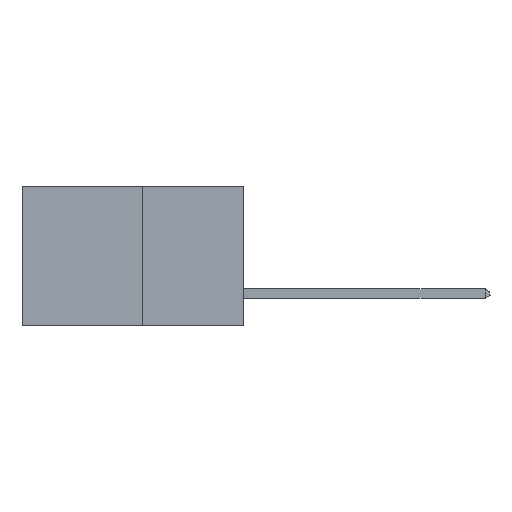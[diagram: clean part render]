
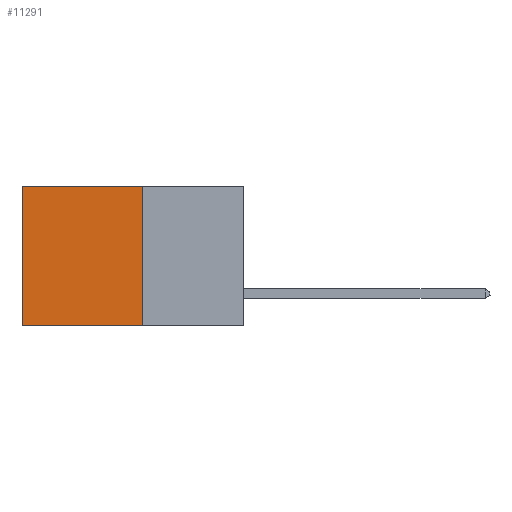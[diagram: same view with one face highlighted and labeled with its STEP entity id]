
A CAD part, left-side view. The second image highlights one B-rep face of the part: STEP entity #11291.
In plain terms, the highlighted planar face has unit normal (-1, 0, 0).
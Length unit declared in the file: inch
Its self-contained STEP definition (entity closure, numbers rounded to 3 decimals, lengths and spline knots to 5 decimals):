
#243 = ORIENTED_EDGE ( 'NONE', *, *, #28271, .T. ) ;
#810 = EDGE_CURVE ( 'NONE', #20137, #5224, #26072, .T. ) ;
#2135 = FACE_OUTER_BOUND ( 'NONE', #20088, .T. ) ;
#4291 = DIRECTION ( 'NONE',  ( 0., 1., 0. ) ) ;
#4607 = ORIENTED_EDGE ( 'NONE', *, *, #16943, .F. ) ;
#5224 = VERTEX_POINT ( 'NONE', #22980 ) ;
#7278 = CARTESIAN_POINT ( 'NONE',  ( 0.277, 0.27, -0.37 ) ) ;
#7582 = CARTESIAN_POINT ( 'NONE',  ( 0.277, 0.59, -0.37 ) ) ;
#8213 = VECTOR ( 'NONE', #23368, 39.37008 ) ;
#8391 = CARTESIAN_POINT ( 'NONE',  ( 0.277, 0.59, -0.37 ) ) ;
#9512 = DIRECTION ( 'NONE',  ( 0., 0., -1. ) ) ;
#9771 = VERTEX_POINT ( 'NONE', #8391 ) ;
#10930 = CARTESIAN_POINT ( 'NONE',  ( 0.277, 0.27, 0. ) ) ;
#11291 = ADVANCED_FACE ( 'NONE', ( #2135 ), #18422, .F. ) ;
#11837 = CARTESIAN_POINT ( 'NONE',  ( 0.277, 0.59, 0. ) ) ;
#14369 = ORIENTED_EDGE ( 'NONE', *, *, #810, .F. ) ;
#15660 = VERTEX_POINT ( 'NONE', #11837 ) ;
#16943 = EDGE_CURVE ( 'NONE', #5224, #9771, #26947, .T. ) ;
#16952 = CARTESIAN_POINT ( 'NONE',  ( 0.277, 0.27, 0. ) ) ;
#18422 = PLANE ( 'NONE',  #28619 ) ;
#18614 = CARTESIAN_POINT ( 'NONE',  ( 0.277, 0.27, -0.37 ) ) ;
#20004 = VECTOR ( 'NONE', #20969, 39.37008 ) ;
#20088 = EDGE_LOOP ( 'NONE', ( #243, #4607, #14369, #20674 ) ) ;
#20137 = VERTEX_POINT ( 'NONE', #16952 ) ;
#20281 = VECTOR ( 'NONE', #27569, 39.37008 ) ;
#20674 = ORIENTED_EDGE ( 'NONE', *, *, #26948, .T. ) ;
#20969 = DIRECTION ( 'NONE',  ( 0., 0., -1. ) ) ;
#22582 = CARTESIAN_POINT ( 'NONE',  ( 0.277, 0.27, -0.37 ) ) ;
#22905 = DIRECTION ( 'NONE',  ( 1., 0., 0. ) ) ;
#22919 = VECTOR ( 'NONE', #4291, 39.37008 ) ;
#22980 = CARTESIAN_POINT ( 'NONE',  ( 0.277, 0.27, -0.37 ) ) ;
#23368 = DIRECTION ( 'NONE',  ( 0., 0., -1. ) ) ;
#26072 = LINE ( 'NONE', #22582, #8213 ) ;
#26668 = LINE ( 'NONE', #7582, #20004 ) ;
#26947 = LINE ( 'NONE', #18614, #20281 ) ;
#26948 = EDGE_CURVE ( 'NONE', #20137, #15660, #28137, .T. ) ;
#27569 = DIRECTION ( 'NONE',  ( 0., 1., 0. ) ) ;
#28137 = LINE ( 'NONE', #10930, #22919 ) ;
#28271 = EDGE_CURVE ( 'NONE', #15660, #9771, #26668, .T. ) ;
#28619 = AXIS2_PLACEMENT_3D ( 'NONE', #7278, #22905, #9512 ) ;
